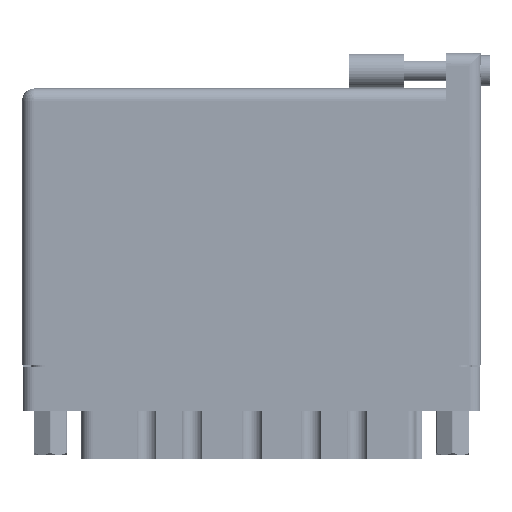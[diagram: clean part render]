
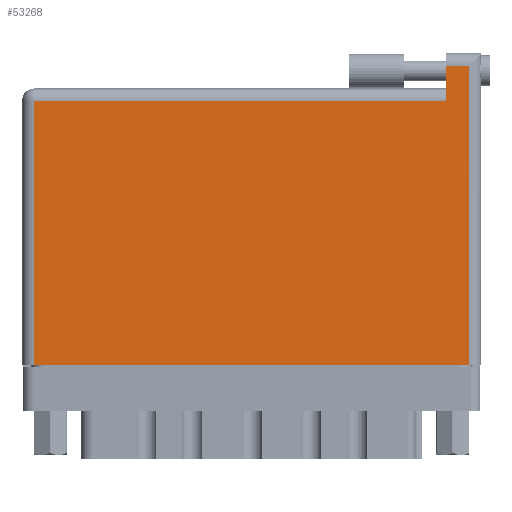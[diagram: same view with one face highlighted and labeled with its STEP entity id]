
A CAD part, front view. The second image highlights one B-rep face of the part: STEP entity #53268.
In plain terms, the highlighted face is planar.
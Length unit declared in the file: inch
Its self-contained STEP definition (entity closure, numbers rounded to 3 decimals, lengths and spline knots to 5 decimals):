
#2588 = LINE ( 'NONE', #43303, #28139 ) ;
#3232 = CARTESIAN_POINT ( 'NONE',  ( 2.403, 1.696, 0. ) ) ;
#4088 = CARTESIAN_POINT ( 'NONE',  ( 0.07, 0., 0. ) ) ;
#6123 = CARTESIAN_POINT ( 'NONE',  ( 2.403, 1.496, 0. ) ) ;
#7114 = ORIENTED_EDGE ( 'NONE', *, *, #10214, .T. ) ;
#7233 = VERTEX_POINT ( 'NONE', #35589 ) ;
#9110 = EDGE_CURVE ( 'NONE', #21740, #24291, #49032, .T. ) ;
#10214 = EDGE_CURVE ( 'NONE', #7233, #43342, #14423, .T. ) ;
#10384 = DIRECTION ( 'NONE',  ( 1., 0., 0. ) ) ;
#13296 = CARTESIAN_POINT ( 'NONE',  ( 2.53, 1.696, 0. ) ) ;
#13312 = VECTOR ( 'NONE', #10384, 39.37008 ) ;
#13690 = AXIS2_PLACEMENT_3D ( 'NONE', #36421, #27259, #22430 ) ;
#14137 = DIRECTION ( 'NONE',  ( -1., 0., 0. ) ) ;
#14423 = LINE ( 'NONE', #17820, #61692 ) ;
#16563 = VERTEX_POINT ( 'NONE', #37809 ) ;
#17369 = PLANE ( 'NONE',  #13690 ) ;
#17820 = CARTESIAN_POINT ( 'NONE',  ( 0.07, 0., 0. ) ) ;
#17920 = ORIENTED_EDGE ( 'NONE', *, *, #30346, .T. ) ;
#21740 = VERTEX_POINT ( 'NONE', #13296 ) ;
#22430 = DIRECTION ( 'NONE',  ( -1., 0., 0. ) ) ;
#23966 = DIRECTION ( 'NONE',  ( 0., 1., 0. ) ) ;
#24291 = VERTEX_POINT ( 'NONE', #3232 ) ;
#24884 = DIRECTION ( 'NONE',  ( 0., -1., 0. ) ) ;
#26134 = LINE ( 'NONE', #33742, #31300 ) ;
#27259 = DIRECTION ( 'NONE',  ( 0., 0., -1. ) ) ;
#28139 = VECTOR ( 'NONE', #24884, 39.37008 ) ;
#30346 = EDGE_CURVE ( 'NONE', #43665, #7233, #34070, .T. ) ;
#30352 = VECTOR ( 'NONE', #14137, 39.37008 ) ;
#30876 = EDGE_LOOP ( 'NONE', ( #36155, #38327, #34521, #52215, #17920, #7114 ) ) ;
#31276 = LINE ( 'NONE', #39058, #13312 ) ;
#31300 = VECTOR ( 'NONE', #23966, 39.37008 ) ;
#33742 = CARTESIAN_POINT ( 'NONE',  ( 2.53, 1.766, 0. ) ) ;
#34070 = LINE ( 'NONE', #42844, #30352 ) ;
#34078 = EDGE_CURVE ( 'NONE', #16563, #21740, #26134, .T. ) ;
#34521 = ORIENTED_EDGE ( 'NONE', *, *, #9110, .T. ) ;
#34842 = FACE_OUTER_BOUND ( 'NONE', #30876, .T. ) ;
#35589 = CARTESIAN_POINT ( 'NONE',  ( 0.07, 1.496, 0. ) ) ;
#36155 = ORIENTED_EDGE ( 'NONE', *, *, #51622, .T. ) ;
#36421 = CARTESIAN_POINT ( 'NONE',  ( 0., 1.566, 0. ) ) ;
#37809 = CARTESIAN_POINT ( 'NONE',  ( 2.53, 0., 0. ) ) ;
#38327 = ORIENTED_EDGE ( 'NONE', *, *, #34078, .T. ) ;
#39058 = CARTESIAN_POINT ( 'NONE',  ( 0., 0., 0. ) ) ;
#42844 = CARTESIAN_POINT ( 'NONE',  ( 0., 1.496, 0. ) ) ;
#43303 = CARTESIAN_POINT ( 'NONE',  ( 2.403, 1.766, 0. ) ) ;
#43342 = VERTEX_POINT ( 'NONE', #4088 ) ;
#43489 = DIRECTION ( 'NONE',  ( -1., 0., 0. ) ) ;
#43665 = VERTEX_POINT ( 'NONE', #6123 ) ;
#47519 = VECTOR ( 'NONE', #43489, 39.37008 ) ;
#48291 = CARTESIAN_POINT ( 'NONE',  ( 0., 1.696, 0. ) ) ;
#49032 = LINE ( 'NONE', #48291, #47519 ) ;
#50341 = EDGE_CURVE ( 'NONE', #24291, #43665, #2588, .T. ) ;
#51622 = EDGE_CURVE ( 'NONE', #43342, #16563, #31276, .T. ) ;
#52215 = ORIENTED_EDGE ( 'NONE', *, *, #50341, .T. ) ;
#53268 = ADVANCED_FACE ( 'NONE', ( #34842 ), #17369, .F. ) ;
#57461 = DIRECTION ( 'NONE',  ( 0., -1., 0. ) ) ;
#61692 = VECTOR ( 'NONE', #57461, 39.37008 ) ;
